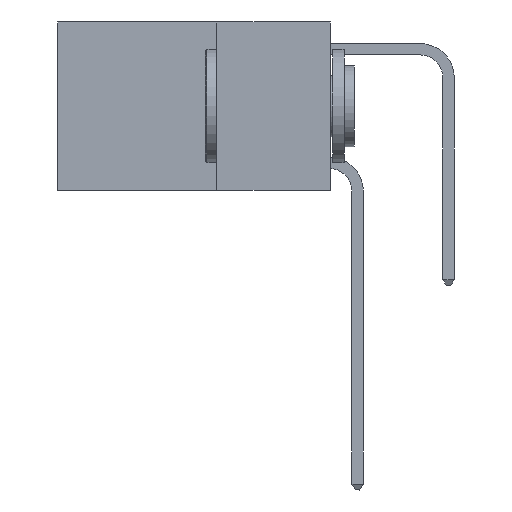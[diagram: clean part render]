
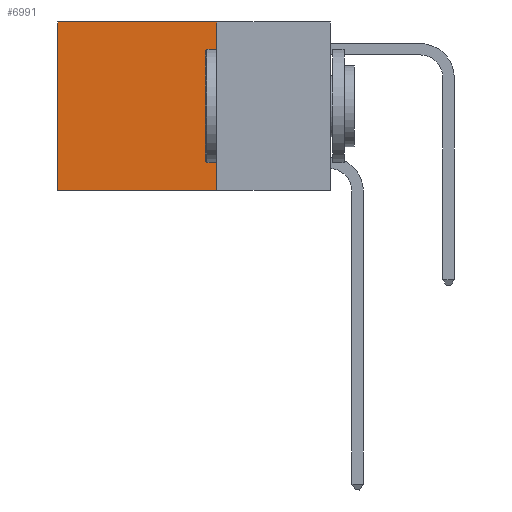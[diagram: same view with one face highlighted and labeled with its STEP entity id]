
A CAD part, left-side view. The second image highlights one B-rep face of the part: STEP entity #6991.
In plain terms, the highlighted planar face has unit normal (-1, 0, 0).
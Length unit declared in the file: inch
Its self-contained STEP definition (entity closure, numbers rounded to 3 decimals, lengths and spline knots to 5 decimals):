
#158 = LINE ( 'NONE', #5187, #15456 ) ;
#1213 = PLANE ( 'NONE',  #10706 ) ;
#1450 = EDGE_LOOP ( 'NONE', ( #1495, #6311, #10380, #2121 ) ) ;
#1495 = ORIENTED_EDGE ( 'NONE', *, *, #12736, .T. ) ;
#1562 = VECTOR ( 'NONE', #13032, 39.37008 ) ;
#1915 = VECTOR ( 'NONE', #8796, 39.37008 ) ;
#2121 = ORIENTED_EDGE ( 'NONE', *, *, #3867, .T. ) ;
#2287 = VERTEX_POINT ( 'NONE', #9731 ) ;
#2457 = EDGE_CURVE ( 'NONE', #6448, #8527, #158, .T. ) ;
#3525 = CARTESIAN_POINT ( 'NONE',  ( 0.2625, 0.6, -0.37 ) ) ;
#3664 = CARTESIAN_POINT ( 'NONE',  ( 0.2625, 0.25, 0. ) ) ;
#3867 = EDGE_CURVE ( 'NONE', #6448, #2287, #15435, .T. ) ;
#5095 = CARTESIAN_POINT ( 'NONE',  ( 0.2625, 0.25, -0.37 ) ) ;
#5187 = CARTESIAN_POINT ( 'NONE',  ( 0.2625, 0.25, 0. ) ) ;
#5823 = LINE ( 'NONE', #14486, #8826 ) ;
#5949 = CARTESIAN_POINT ( 'NONE',  ( 0.2625, 0.25, 0. ) ) ;
#6238 = DIRECTION ( 'NONE',  ( 0., 0., -1. ) ) ;
#6311 = ORIENTED_EDGE ( 'NONE', *, *, #10022, .F. ) ;
#6448 = VERTEX_POINT ( 'NONE', #5949 ) ;
#6991 = ADVANCED_FACE ( 'NONE', ( #7558 ), #1213, .F. ) ;
#7558 = FACE_OUTER_BOUND ( 'NONE', #1450, .T. ) ;
#7722 = LINE ( 'NONE', #11511, #1915 ) ;
#7911 = DIRECTION ( 'NONE',  ( 0., 0., -1. ) ) ;
#8086 = CARTESIAN_POINT ( 'NONE',  ( 0.2625, 0.25, 0. ) ) ;
#8527 = VERTEX_POINT ( 'NONE', #5095 ) ;
#8796 = DIRECTION ( 'NONE',  ( 0., 1., 0. ) ) ;
#8826 = VECTOR ( 'NONE', #12995, 39.37008 ) ;
#9731 = CARTESIAN_POINT ( 'NONE',  ( 0.2625, 0.6, 0. ) ) ;
#10022 = EDGE_CURVE ( 'NONE', #8527, #10769, #7722, .T. ) ;
#10380 = ORIENTED_EDGE ( 'NONE', *, *, #2457, .F. ) ;
#10706 = AXIS2_PLACEMENT_3D ( 'NONE', #3664, #12500, #6238 ) ;
#10769 = VERTEX_POINT ( 'NONE', #3525 ) ;
#11511 = CARTESIAN_POINT ( 'NONE',  ( 0.2625, 0.25, -0.37 ) ) ;
#12500 = DIRECTION ( 'NONE',  ( 1., 0., 0. ) ) ;
#12736 = EDGE_CURVE ( 'NONE', #2287, #10769, #5823, .T. ) ;
#12995 = DIRECTION ( 'NONE',  ( 0., 0., -1. ) ) ;
#13032 = DIRECTION ( 'NONE',  ( 0., 1., 0. ) ) ;
#14486 = CARTESIAN_POINT ( 'NONE',  ( 0.2625, 0.6, 0. ) ) ;
#15435 = LINE ( 'NONE', #8086, #1562 ) ;
#15456 = VECTOR ( 'NONE', #7911, 39.37008 ) ;
